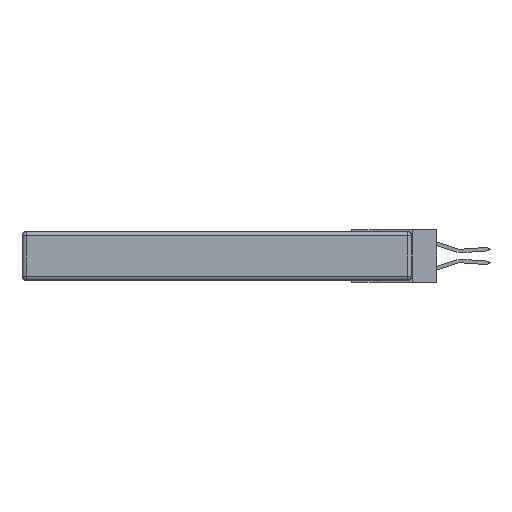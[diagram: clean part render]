
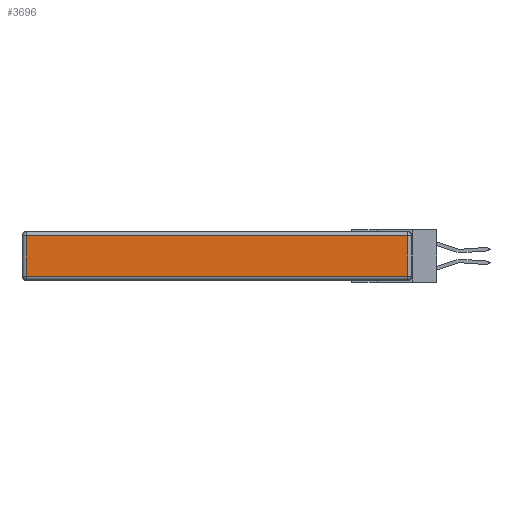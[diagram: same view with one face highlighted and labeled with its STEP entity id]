
A CAD part, left-side view. The second image highlights one B-rep face of the part: STEP entity #3696.
In plain terms, the highlighted planar face has unit normal (-1, 0, 0).
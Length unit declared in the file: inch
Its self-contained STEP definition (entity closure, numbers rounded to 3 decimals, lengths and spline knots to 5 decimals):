
#2947 = ORIENTED_EDGE ( 'NONE', *, *, #18432, .T. ) ;
#3097 = LINE ( 'NONE', #15515, #20291 ) ;
#3228 = PLANE ( 'NONE',  #22697 ) ;
#3696 = ADVANCED_FACE ( 'NONE', ( #15797 ), #3228, .T. ) ;
#5280 = CARTESIAN_POINT ( 'NONE',  ( 0., 2.72, -0.03 ) ) ;
#5413 = VERTEX_POINT ( 'NONE', #5280 ) ;
#6052 = ORIENTED_EDGE ( 'NONE', *, *, #15337, .T. ) ;
#7722 = DIRECTION ( 'NONE',  ( -1., 0., 0. ) ) ;
#7918 = LINE ( 'NONE', #11092, #13597 ) ;
#8354 = DIRECTION ( 'NONE',  ( 0., 0., -1. ) ) ;
#9250 = VECTOR ( 'NONE', #8354, 39.37008 ) ;
#9527 = ORIENTED_EDGE ( 'NONE', *, *, #10523, .T. ) ;
#10045 = VERTEX_POINT ( 'NONE', #27363 ) ;
#10523 = EDGE_CURVE ( 'NONE', #10045, #11192, #7918, .T. ) ;
#10821 = CARTESIAN_POINT ( 'NONE',  ( 0., 2.72, -0.343 ) ) ;
#11003 = LINE ( 'NONE', #10821, #9250 ) ;
#11092 = CARTESIAN_POINT ( 'NONE',  ( 0., 0., -0.313 ) ) ;
#11192 = VERTEX_POINT ( 'NONE', #14868 ) ;
#13205 = DIRECTION ( 'NONE',  ( 0., 1., 0. ) ) ;
#13597 = VECTOR ( 'NONE', #27015, 39.37008 ) ;
#14868 = CARTESIAN_POINT ( 'NONE',  ( 0., 0.03, -0.313 ) ) ;
#15142 = DIRECTION ( 'NONE',  ( 0., 0., 1. ) ) ;
#15337 = EDGE_CURVE ( 'NONE', #5413, #10045, #11003, .T. ) ;
#15493 = EDGE_LOOP ( 'NONE', ( #9527, #2947, #19514, #6052 ) ) ;
#15515 = CARTESIAN_POINT ( 'NONE',  ( 0., 0.03, -0.343 ) ) ;
#15797 = FACE_OUTER_BOUND ( 'NONE', #15493, .T. ) ;
#17349 = CARTESIAN_POINT ( 'NONE',  ( 0., 0.03, -0.03 ) ) ;
#17533 = CARTESIAN_POINT ( 'NONE',  ( 0., 2.75, -0.03 ) ) ;
#18432 = EDGE_CURVE ( 'NONE', #11192, #26690, #3097, .T. ) ;
#19514 = ORIENTED_EDGE ( 'NONE', *, *, #20331, .T. ) ;
#20291 = VECTOR ( 'NONE', #15142, 39.37008 ) ;
#20331 = EDGE_CURVE ( 'NONE', #26690, #5413, #24096, .T. ) ;
#20986 = DIRECTION ( 'NONE',  ( 0., 0., 1. ) ) ;
#21175 = CARTESIAN_POINT ( 'NONE',  ( 0., 0., -0.343 ) ) ;
#22697 = AXIS2_PLACEMENT_3D ( 'NONE', #21175, #7722, #20986 ) ;
#24096 = LINE ( 'NONE', #17533, #28652 ) ;
#26690 = VERTEX_POINT ( 'NONE', #17349 ) ;
#27015 = DIRECTION ( 'NONE',  ( 0., -1., 0. ) ) ;
#27363 = CARTESIAN_POINT ( 'NONE',  ( 0., 2.72, -0.313 ) ) ;
#28652 = VECTOR ( 'NONE', #13205, 39.37008 ) ;
